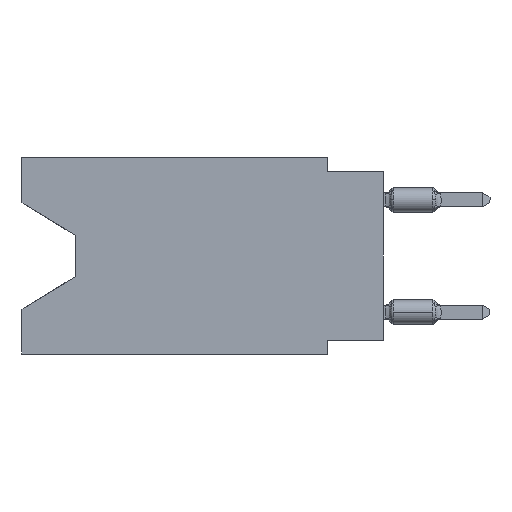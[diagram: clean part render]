
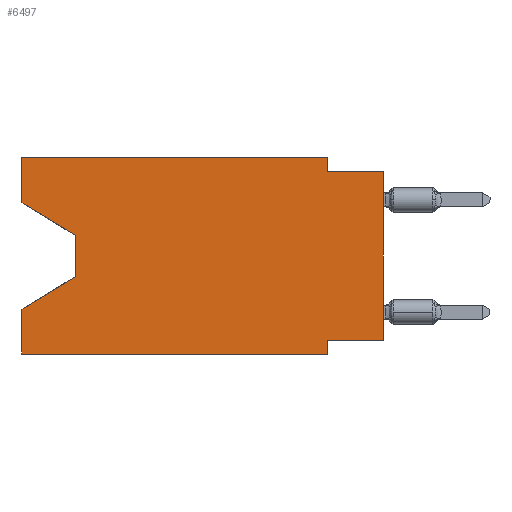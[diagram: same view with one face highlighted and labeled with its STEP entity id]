
A CAD part, left-side view. The second image highlights one B-rep face of the part: STEP entity #6497.
In plain terms, the highlighted planar face has unit normal (-1, 0, 0).
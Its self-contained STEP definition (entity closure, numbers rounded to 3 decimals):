
#48 = VERTEX_POINT ( 'NONE', #4199 ) ;
#257 = EDGE_CURVE ( 'NONE', #1758, #5720, #3709, .T. ) ;
#609 = CARTESIAN_POINT ( 'NONE',  ( 0., 13.97, -5.385 ) ) ;
#614 = DIRECTION ( 'NONE',  ( 0., 0., -1. ) ) ;
#639 = DIRECTION ( 'NONE',  ( 0., 0., -1. ) ) ;
#642 = CARTESIAN_POINT ( 'NONE',  ( 0., 0., 0. ) ) ;
#883 = ORIENTED_EDGE ( 'NONE', *, *, #7530, .T. ) ;
#1053 = CARTESIAN_POINT ( 'NONE',  ( 0., 16.383, 0. ) ) ;
#1056 = ORIENTED_EDGE ( 'NONE', *, *, #1847, .T. ) ;
#1265 = VERTEX_POINT ( 'NONE', #2549 ) ;
#1758 = VERTEX_POINT ( 'NONE', #12908 ) ;
#1847 = EDGE_CURVE ( 'NONE', #12449, #5187, #6620, .T. ) ;
#2001 = VERTEX_POINT ( 'NONE', #12044 ) ;
#2108 = EDGE_CURVE ( 'NONE', #13642, #10923, #12244, .T. ) ;
#2153 = LINE ( 'NONE', #1053, #13033 ) ;
#2363 = EDGE_CURVE ( 'NONE', #13642, #12778, #10707, .T. ) ;
#2405 = LINE ( 'NONE', #12914, #9989 ) ;
#2412 = ORIENTED_EDGE ( 'NONE', *, *, #5739, .F. ) ;
#2439 = VECTOR ( 'NONE', #12157, 1000. ) ;
#2542 = DIRECTION ( 'NONE',  ( 0., 0.855, -0.519 ) ) ;
#2549 = CARTESIAN_POINT ( 'NONE',  ( 0., 2.54, -0.635 ) ) ;
#2611 = ORIENTED_EDGE ( 'NONE', *, *, #6800, .F. ) ;
#2715 = VECTOR ( 'NONE', #8007, 1000. ) ;
#2768 = DIRECTION ( 'NONE',  ( 0., 0., 1. ) ) ;
#3031 = CARTESIAN_POINT ( 'NONE',  ( 0., 0., -8.255 ) ) ;
#3099 = DIRECTION ( 'NONE',  ( 0., -1., 0. ) ) ;
#3321 = VECTOR ( 'NONE', #8377, 1000. ) ;
#3343 = EDGE_LOOP ( 'NONE', ( #3888, #1056, #883, #5623, #12684, #9336, #4174, #6934, #9838, #2412, #2611, #4868 ) ) ;
#3709 = LINE ( 'NONE', #7935, #2439 ) ;
#3715 = LINE ( 'NONE', #7103, #2715 ) ;
#3720 = EDGE_CURVE ( 'NONE', #48, #12449, #7206, .T. ) ;
#3888 = ORIENTED_EDGE ( 'NONE', *, *, #3720, .T. ) ;
#4033 = AXIS2_PLACEMENT_3D ( 'NONE', #4893, #12228, #13188 ) ;
#4174 = ORIENTED_EDGE ( 'NONE', *, *, #2363, .F. ) ;
#4199 = CARTESIAN_POINT ( 'NONE',  ( 0., 16.383, -2.038 ) ) ;
#4725 = LINE ( 'NONE', #7651, #6211 ) ;
#4816 = CARTESIAN_POINT ( 'NONE',  ( 0., 13.97, -3.505 ) ) ;
#4868 = ORIENTED_EDGE ( 'NONE', *, *, #12639, .F. ) ;
#4893 = CARTESIAN_POINT ( 'NONE',  ( 0., 16.383, 0. ) ) ;
#5187 = VERTEX_POINT ( 'NONE', #609 ) ;
#5352 = VECTOR ( 'NONE', #639, 1000. ) ;
#5623 = ORIENTED_EDGE ( 'NONE', *, *, #10077, .F. ) ;
#5720 = VERTEX_POINT ( 'NONE', #10243 ) ;
#5739 = EDGE_CURVE ( 'NONE', #9757, #1265, #9411, .T. ) ;
#5940 = LINE ( 'NONE', #10098, #5352 ) ;
#6165 = CARTESIAN_POINT ( 'NONE',  ( 0., 16.383, -2.038 ) ) ;
#6211 = VECTOR ( 'NONE', #12906, 1000. ) ;
#6497 = ADVANCED_FACE ( 'NONE', ( #9049 ), #9111, .F. ) ;
#6620 = LINE ( 'NONE', #4816, #13636 ) ;
#6640 = CARTESIAN_POINT ( 'NONE',  ( 0., 2.54, -8.255 ) ) ;
#6800 = EDGE_CURVE ( 'NONE', #10725, #9757, #4725, .T. ) ;
#6934 = ORIENTED_EDGE ( 'NONE', *, *, #2108, .T. ) ;
#7103 = CARTESIAN_POINT ( 'NONE',  ( 0., 16.383, 0. ) ) ;
#7206 = LINE ( 'NONE', #6165, #10721 ) ;
#7251 = DIRECTION ( 'NONE',  ( 0., 1., 0. ) ) ;
#7397 = VECTOR ( 'NONE', #7251, 1000. ) ;
#7416 = EDGE_CURVE ( 'NONE', #12778, #5720, #5940, .T. ) ;
#7530 = EDGE_CURVE ( 'NONE', #5187, #2001, #2405, .T. ) ;
#7651 = CARTESIAN_POINT ( 'NONE',  ( 0., 16.383, 0. ) ) ;
#7935 = CARTESIAN_POINT ( 'NONE',  ( 0., 16.383, -8.89 ) ) ;
#8007 = DIRECTION ( 'NONE',  ( 0., 0., 1. ) ) ;
#8377 = DIRECTION ( 'NONE',  ( 0., 0., -1. ) ) ;
#9049 = FACE_OUTER_BOUND ( 'NONE', #3343, .T. ) ;
#9081 = CARTESIAN_POINT ( 'NONE',  ( 0., 0., -8.255 ) ) ;
#9111 = PLANE ( 'NONE',  #4033 ) ;
#9336 = ORIENTED_EDGE ( 'NONE', *, *, #7416, .F. ) ;
#9411 = LINE ( 'NONE', #12663, #3321 ) ;
#9453 = VECTOR ( 'NONE', #2768, 1000. ) ;
#9535 = CARTESIAN_POINT ( 'NONE',  ( 0., 2.54, 0. ) ) ;
#9733 = EDGE_CURVE ( 'NONE', #1265, #10923, #10706, .T. ) ;
#9757 = VERTEX_POINT ( 'NONE', #9535 ) ;
#9838 = ORIENTED_EDGE ( 'NONE', *, *, #9733, .F. ) ;
#9968 = CARTESIAN_POINT ( 'NONE',  ( 0., 13.97, -3.505 ) ) ;
#9989 = VECTOR ( 'NONE', #2542, 1000. ) ;
#10077 = EDGE_CURVE ( 'NONE', #1758, #2001, #3715, .T. ) ;
#10098 = CARTESIAN_POINT ( 'NONE',  ( 0., 2.54, -8.89 ) ) ;
#10243 = CARTESIAN_POINT ( 'NONE',  ( 0., 2.54, -8.89 ) ) ;
#10385 = DIRECTION ( 'NONE',  ( 0., -0.855, -0.519 ) ) ;
#10644 = VECTOR ( 'NONE', #3099, 1000. ) ;
#10706 = LINE ( 'NONE', #12792, #10644 ) ;
#10707 = LINE ( 'NONE', #3031, #7397 ) ;
#10721 = VECTOR ( 'NONE', #10385, 1000. ) ;
#10725 = VERTEX_POINT ( 'NONE', #12045 ) ;
#10923 = VERTEX_POINT ( 'NONE', #13538 ) ;
#11685 = DIRECTION ( 'NONE',  ( 0., 0., 1. ) ) ;
#12044 = CARTESIAN_POINT ( 'NONE',  ( 0., 16.383, -6.852 ) ) ;
#12045 = CARTESIAN_POINT ( 'NONE',  ( 0., 16.383, 0. ) ) ;
#12157 = DIRECTION ( 'NONE',  ( 0., -1., 0. ) ) ;
#12228 = DIRECTION ( 'NONE',  ( 1., 0., 0. ) ) ;
#12244 = LINE ( 'NONE', #642, #9453 ) ;
#12449 = VERTEX_POINT ( 'NONE', #9968 ) ;
#12639 = EDGE_CURVE ( 'NONE', #48, #10725, #2153, .T. ) ;
#12663 = CARTESIAN_POINT ( 'NONE',  ( 0., 2.54, 0. ) ) ;
#12684 = ORIENTED_EDGE ( 'NONE', *, *, #257, .T. ) ;
#12778 = VERTEX_POINT ( 'NONE', #6640 ) ;
#12792 = CARTESIAN_POINT ( 'NONE',  ( 0., 0., -0.635 ) ) ;
#12906 = DIRECTION ( 'NONE',  ( 0., -1., 0. ) ) ;
#12908 = CARTESIAN_POINT ( 'NONE',  ( 0., 16.383, -8.89 ) ) ;
#12914 = CARTESIAN_POINT ( 'NONE',  ( 0., 13.97, -5.385 ) ) ;
#13033 = VECTOR ( 'NONE', #11685, 1000. ) ;
#13188 = DIRECTION ( 'NONE',  ( 0., 0., -1. ) ) ;
#13538 = CARTESIAN_POINT ( 'NONE',  ( 0., 0., -0.635 ) ) ;
#13636 = VECTOR ( 'NONE', #614, 1000. ) ;
#13642 = VERTEX_POINT ( 'NONE', #9081 ) ;
